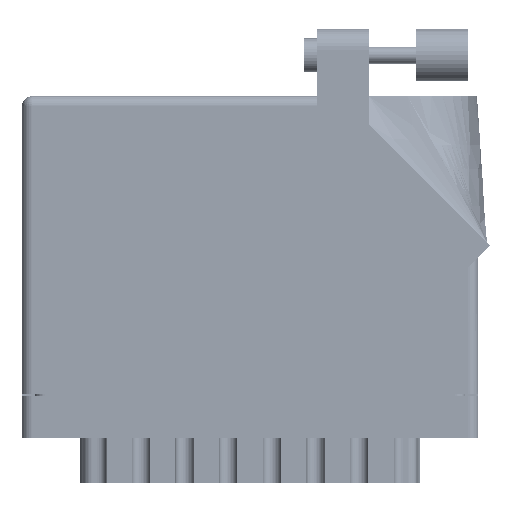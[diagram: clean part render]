
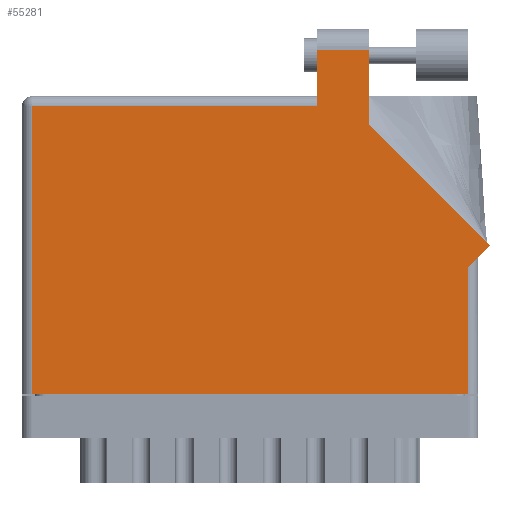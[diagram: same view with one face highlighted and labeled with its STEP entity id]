
A CAD part, front view. The second image highlights one B-rep face of the part: STEP entity #55281.
In plain terms, the highlighted face is planar.
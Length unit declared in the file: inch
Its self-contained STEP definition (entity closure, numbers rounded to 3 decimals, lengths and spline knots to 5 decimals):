
#141 = VECTOR ( 'NONE', #68062, 39.37008 ) ;
#1661 = CARTESIAN_POINT ( 'NONE',  ( 2.656, 0.753, 0. ) ) ;
#1807 = EDGE_CURVE ( 'NONE', #20348, #9801, #3185, .T. ) ;
#3185 = LINE ( 'NONE', #71511, #30881 ) ;
#4669 = EDGE_CURVE ( 'NONE', #61582, #51054, #49023, .T. ) ;
#5674 = DIRECTION ( 'NONE',  ( -1., 0., 0. ) ) ;
#6466 = FACE_OUTER_BOUND ( 'NONE', #44404, .T. ) ;
#8747 = DIRECTION ( 'NONE',  ( -1., 0., 0. ) ) ;
#8830 = VERTEX_POINT ( 'NONE', #76526 ) ;
#9214 = ORIENTED_EDGE ( 'NONE', *, *, #48413, .T. ) ;
#9588 = VECTOR ( 'NONE', #27651, 39.37008 ) ;
#9801 = VERTEX_POINT ( 'NONE', #1661 ) ;
#17088 = EDGE_CURVE ( 'NONE', #25402, #20348, #60226, .T. ) ;
#17426 = CARTESIAN_POINT ( 'NONE',  ( 1.758, 2.05, 0. ) ) ;
#19444 = DIRECTION ( 'NONE',  ( -1., 0., 0. ) ) ;
#20018 = CARTESIAN_POINT ( 'NONE',  ( 2.718, 0.815, 0. ) ) ;
#20348 = VERTEX_POINT ( 'NONE', #33563 ) ;
#24422 = CARTESIAN_POINT ( 'NONE',  ( 0.062, 0., 0. ) ) ;
#24462 = ORIENTED_EDGE ( 'NONE', *, *, #27757, .T. ) ;
#25293 = LINE ( 'NONE', #27155, #9588 ) ;
#25402 = VERTEX_POINT ( 'NONE', #25965 ) ;
#25965 = CARTESIAN_POINT ( 'NONE',  ( 0.062, 0., 0. ) ) ;
#26948 = VECTOR ( 'NONE', #73224, 39.37008 ) ;
#27155 = CARTESIAN_POINT ( 'NONE',  ( 2.78871, 0.88571, 0. ) ) ;
#27651 = DIRECTION ( 'NONE',  ( -0.707, 0.707, 0. ) ) ;
#27757 = EDGE_CURVE ( 'NONE', #59054, #68263, #44107, .T. ) ;
#29149 = DIRECTION ( 'NONE',  ( 0., 0., -1. ) ) ;
#30881 = VECTOR ( 'NONE', #66888, 39.37008 ) ;
#32100 = VECTOR ( 'NONE', #19444, 39.37008 ) ;
#32488 = ORIENTED_EDGE ( 'NONE', *, *, #1807, .T. ) ;
#33449 = CARTESIAN_POINT ( 'NONE',  ( 2.065, 2.05, 0. ) ) ;
#33563 = CARTESIAN_POINT ( 'NONE',  ( 2.656, 0., 0. ) ) ;
#34190 = VECTOR ( 'NONE', #8747, 39.37008 ) ;
#35192 = ORIENTED_EDGE ( 'NONE', *, *, #63257, .T. ) ;
#38438 = CARTESIAN_POINT ( 'NONE',  ( 1.758, 2.05, 0. ) ) ;
#41524 = CARTESIAN_POINT ( 'NONE',  ( 0., 1.775, 0. ) ) ;
#42324 = LINE ( 'NONE', #73680, #32100 ) ;
#44107 = LINE ( 'NONE', #61278, #46861 ) ;
#44404 = EDGE_LOOP ( 'NONE', ( #58393, #54726, #24462, #9214, #35192, #46387, #32488, #56619, #56206 ) ) ;
#45467 = DIRECTION ( 'NONE',  ( 0., 1., 0. ) ) ;
#46282 = LINE ( 'NONE', #38438, #34190 ) ;
#46387 = ORIENTED_EDGE ( 'NONE', *, *, #17088, .T. ) ;
#46861 = VECTOR ( 'NONE', #66735, 39.37008 ) ;
#47069 = EDGE_CURVE ( 'NONE', #51054, #59054, #46282, .T. ) ;
#47504 = AXIS2_PLACEMENT_3D ( 'NONE', #41524, #29149, #5674 ) ;
#48413 = EDGE_CURVE ( 'NONE', #68263, #55789, #42324, .T. ) ;
#49023 = LINE ( 'NONE', #57108, #61965 ) ;
#51054 = VERTEX_POINT ( 'NONE', #33449 ) ;
#52768 = LINE ( 'NONE', #20018, #141 ) ;
#54726 = ORIENTED_EDGE ( 'NONE', *, *, #47069, .T. ) ;
#55281 = ADVANCED_FACE ( 'NONE', ( #6466 ), #70507, .F. ) ;
#55789 = VERTEX_POINT ( 'NONE', #59242 ) ;
#56206 = ORIENTED_EDGE ( 'NONE', *, *, #62297, .T. ) ;
#56619 = ORIENTED_EDGE ( 'NONE', *, *, #74156, .T. ) ;
#57108 = CARTESIAN_POINT ( 'NONE',  ( 2.065, 1.60942, 0. ) ) ;
#57464 = LINE ( 'NONE', #24422, #60188 ) ;
#58393 = ORIENTED_EDGE ( 'NONE', *, *, #4669, .T. ) ;
#59054 = VERTEX_POINT ( 'NONE', #17426 ) ;
#59242 = CARTESIAN_POINT ( 'NONE',  ( 0.062, 1.713, 0. ) ) ;
#59796 = DIRECTION ( 'NONE',  ( 0., -1., 0. ) ) ;
#60188 = VECTOR ( 'NONE', #59796, 39.37008 ) ;
#60226 = LINE ( 'NONE', #66781, #26948 ) ;
#61278 = CARTESIAN_POINT ( 'NONE',  ( 1.758, 1.775, 0. ) ) ;
#61582 = VERTEX_POINT ( 'NONE', #62194 ) ;
#61965 = VECTOR ( 'NONE', #45467, 39.37008 ) ;
#62194 = CARTESIAN_POINT ( 'NONE',  ( 2.065, 1.60942, 0. ) ) ;
#62297 = EDGE_CURVE ( 'NONE', #8830, #61582, #25293, .T. ) ;
#63257 = EDGE_CURVE ( 'NONE', #55789, #25402, #57464, .T. ) ;
#66735 = DIRECTION ( 'NONE',  ( 0., -1., 0. ) ) ;
#66781 = CARTESIAN_POINT ( 'NONE',  ( 0., 0., 0. ) ) ;
#66888 = DIRECTION ( 'NONE',  ( 0., 1., 0. ) ) ;
#68062 = DIRECTION ( 'NONE',  ( 0.707, 0.707, 0. ) ) ;
#68263 = VERTEX_POINT ( 'NONE', #69155 ) ;
#69155 = CARTESIAN_POINT ( 'NONE',  ( 1.758, 1.713, 0. ) ) ;
#70507 = PLANE ( 'NONE',  #47504 ) ;
#71511 = CARTESIAN_POINT ( 'NONE',  ( 2.656, 0.815, 0. ) ) ;
#73224 = DIRECTION ( 'NONE',  ( 1., 0., 0. ) ) ;
#73680 = CARTESIAN_POINT ( 'NONE',  ( 0., 1.713, 0. ) ) ;
#74156 = EDGE_CURVE ( 'NONE', #9801, #8830, #52768, .T. ) ;
#76526 = CARTESIAN_POINT ( 'NONE',  ( 2.78871, 0.88571, 0. ) ) ;
